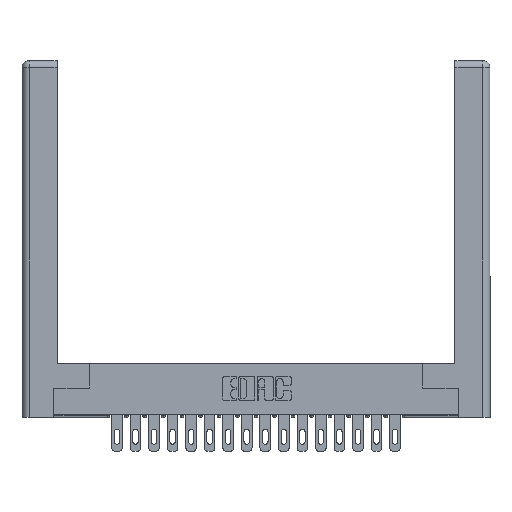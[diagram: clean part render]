
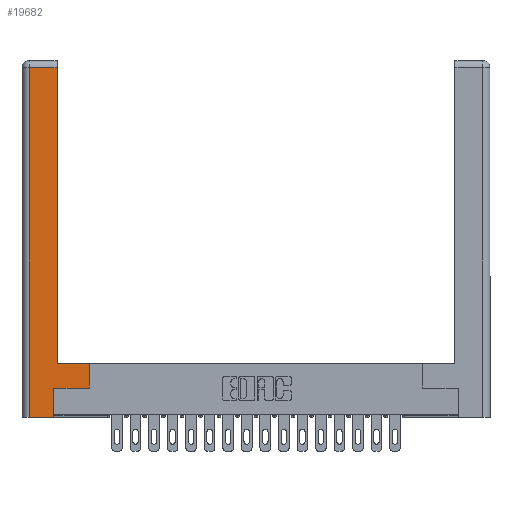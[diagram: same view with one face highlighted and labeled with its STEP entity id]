
A CAD part, top view. The second image highlights one B-rep face of the part: STEP entity #19682.
In plain terms, the highlighted planar face has unit normal (0, 0, 1).
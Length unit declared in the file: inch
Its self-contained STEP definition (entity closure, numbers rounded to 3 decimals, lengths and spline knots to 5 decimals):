
#248 = CARTESIAN_POINT ( 'NONE',  ( 0., 0., 0. ) ) ;
#612 = CARTESIAN_POINT ( 'NONE',  ( 0.265, 0.245, 0. ) ) ;
#834 = ORIENTED_EDGE ( 'NONE', *, *, #20628, .T. ) ;
#1078 = DIRECTION ( 'NONE',  ( 0., -1., 0. ) ) ;
#1331 = ORIENTED_EDGE ( 'NONE', *, *, #2373, .T. ) ;
#1646 = VERTEX_POINT ( 'NONE', #21074 ) ;
#1751 = ORIENTED_EDGE ( 'NONE', *, *, #21483, .T. ) ;
#2176 = PLANE ( 'NONE',  #22071 ) ;
#2238 = ORIENTED_EDGE ( 'NONE', *, *, #17620, .T. ) ;
#2239 = VECTOR ( 'NONE', #13171, 39.37008 ) ;
#2271 = CARTESIAN_POINT ( 'NONE',  ( 0.0615, 2.94, 0. ) ) ;
#2373 = EDGE_CURVE ( 'NONE', #15327, #8625, #8935, .T. ) ;
#2478 = VECTOR ( 'NONE', #6037, 39.37008 ) ;
#2556 = CARTESIAN_POINT ( 'NONE',  ( 0.565, 0.245, 0. ) ) ;
#2798 = LINE ( 'NONE', #2271, #20728 ) ;
#3222 = EDGE_CURVE ( 'NONE', #14654, #15327, #21836, .T. ) ;
#3468 = LINE ( 'NONE', #22124, #21968 ) ;
#4060 = DIRECTION ( 'NONE',  ( -1., 0., 0. ) ) ;
#4477 = VERTEX_POINT ( 'NONE', #8294 ) ;
#4488 = CARTESIAN_POINT ( 'NONE',  ( 0.295, 0.45, 0. ) ) ;
#4661 = LINE ( 'NONE', #17460, #22899 ) ;
#5150 = EDGE_CURVE ( 'NONE', #16659, #4477, #4661, .T. ) ;
#5621 = CARTESIAN_POINT ( 'NONE',  ( 0.0615, 2.94, 0. ) ) ;
#6037 = DIRECTION ( 'NONE',  ( 0., 1., 0. ) ) ;
#6073 = ORIENTED_EDGE ( 'NONE', *, *, #3222, .T. ) ;
#6805 = VECTOR ( 'NONE', #20088, 39.37008 ) ;
#7513 = DIRECTION ( 'NONE',  ( 1., 0., 0. ) ) ;
#7787 = CARTESIAN_POINT ( 'NONE',  ( 0.295, 0.45, 0. ) ) ;
#7858 = CARTESIAN_POINT ( 'NONE',  ( 0.295, 2.94, 0. ) ) ;
#8294 = CARTESIAN_POINT ( 'NONE',  ( 0.0615, 0., 0. ) ) ;
#8305 = LINE ( 'NONE', #612, #2478 ) ;
#8625 = VERTEX_POINT ( 'NONE', #7858 ) ;
#8935 = LINE ( 'NONE', #20942, #16544 ) ;
#9730 = DIRECTION ( 'NONE',  ( 1., 0., 0. ) ) ;
#10869 = FACE_OUTER_BOUND ( 'NONE', #19855, .T. ) ;
#11047 = CARTESIAN_POINT ( 'NONE',  ( 0.565, 0.45, 0. ) ) ;
#11792 = EDGE_CURVE ( 'NONE', #8625, #16659, #2798, .T. ) ;
#13171 = DIRECTION ( 'NONE',  ( -1., 0., 0. ) ) ;
#13804 = CARTESIAN_POINT ( 'NONE',  ( 0.265, 0., 0. ) ) ;
#14355 = EDGE_CURVE ( 'NONE', #21650, #14654, #20285, .T. ) ;
#14654 = VERTEX_POINT ( 'NONE', #21178 ) ;
#14780 = DIRECTION ( 'NONE',  ( 0., 0., -1. ) ) ;
#15327 = VERTEX_POINT ( 'NONE', #7787 ) ;
#15767 = ORIENTED_EDGE ( 'NONE', *, *, #5150, .T. ) ;
#16544 = VECTOR ( 'NONE', #22808, 39.37008 ) ;
#16659 = VERTEX_POINT ( 'NONE', #5621 ) ;
#16815 = CARTESIAN_POINT ( 'NONE',  ( 0.265, 0., 0. ) ) ;
#17121 = VECTOR ( 'NONE', #9730, 39.37008 ) ;
#17460 = CARTESIAN_POINT ( 'NONE',  ( 0.0615, 0., 0. ) ) ;
#17620 = EDGE_CURVE ( 'NONE', #4477, #21772, #23038, .T. ) ;
#18045 = DIRECTION ( 'NONE',  ( -1., 0., 0. ) ) ;
#19682 = ADVANCED_FACE ( 'NONE', ( #10869 ), #2176, .F. ) ;
#19855 = EDGE_LOOP ( 'NONE', ( #1331, #22678, #15767, #2238, #834, #1751, #21525, #6073 ) ) ;
#20088 = DIRECTION ( 'NONE',  ( 0., 1., 0. ) ) ;
#20285 = LINE ( 'NONE', #11047, #6805 ) ;
#20628 = EDGE_CURVE ( 'NONE', #21772, #1646, #8305, .T. ) ;
#20728 = VECTOR ( 'NONE', #4060, 39.37008 ) ;
#20942 = CARTESIAN_POINT ( 'NONE',  ( 0.295, 3., 0. ) ) ;
#21074 = CARTESIAN_POINT ( 'NONE',  ( 0.265, 0.245, 0. ) ) ;
#21178 = CARTESIAN_POINT ( 'NONE',  ( 0.565, 0.45, 0. ) ) ;
#21483 = EDGE_CURVE ( 'NONE', #1646, #21650, #3468, .T. ) ;
#21525 = ORIENTED_EDGE ( 'NONE', *, *, #14355, .T. ) ;
#21650 = VERTEX_POINT ( 'NONE', #2556 ) ;
#21772 = VERTEX_POINT ( 'NONE', #13804 ) ;
#21836 = LINE ( 'NONE', #4488, #2239 ) ;
#21968 = VECTOR ( 'NONE', #7513, 39.37008 ) ;
#22071 = AXIS2_PLACEMENT_3D ( 'NONE', #248, #14780, #18045 ) ;
#22124 = CARTESIAN_POINT ( 'NONE',  ( 0.565, 0.245, 0. ) ) ;
#22678 = ORIENTED_EDGE ( 'NONE', *, *, #11792, .T. ) ;
#22808 = DIRECTION ( 'NONE',  ( 0., 1., 0. ) ) ;
#22899 = VECTOR ( 'NONE', #1078, 39.37008 ) ;
#23038 = LINE ( 'NONE', #16815, #17121 ) ;
